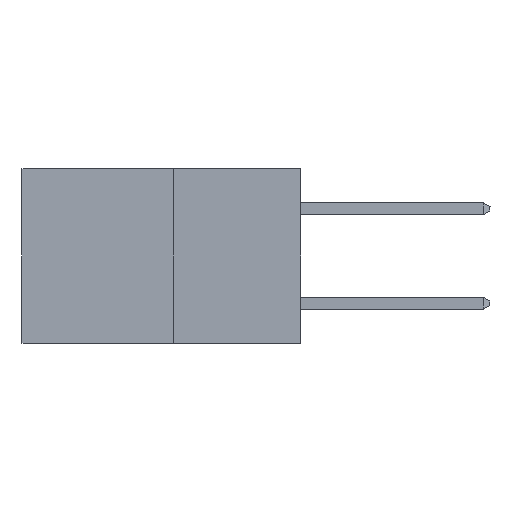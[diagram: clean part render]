
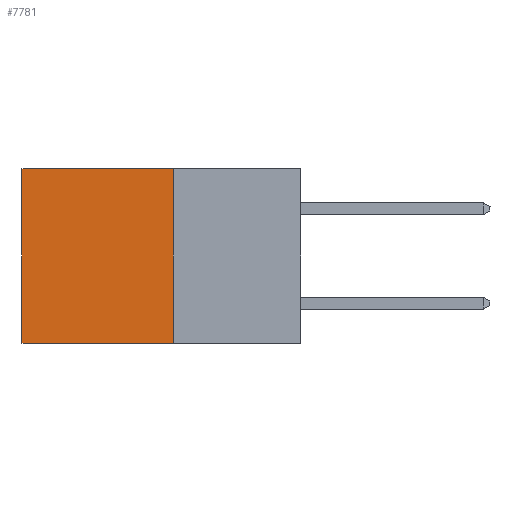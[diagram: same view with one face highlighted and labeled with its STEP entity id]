
A CAD part, left-side view. The second image highlights one B-rep face of the part: STEP entity #7781.
In plain terms, the highlighted planar face has unit normal (-1, 0, 0).
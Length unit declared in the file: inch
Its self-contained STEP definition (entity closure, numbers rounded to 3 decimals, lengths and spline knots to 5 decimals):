
#81 = EDGE_CURVE ( 'NONE', #2081, #1824, #5526, .T. ) ;
#1258 = DIRECTION ( 'NONE',  ( 0., 1., 0. ) ) ;
#1311 = LINE ( 'NONE', #8585, #3317 ) ;
#1323 = EDGE_CURVE ( 'NONE', #1824, #3009, #1311, .T. ) ;
#1560 = ORIENTED_EDGE ( 'NONE', *, *, #2377, .T. ) ;
#1824 = VERTEX_POINT ( 'NONE', #7025 ) ;
#1827 = CARTESIAN_POINT ( 'NONE',  ( 0.277, 0.59, -0.37 ) ) ;
#2081 = VERTEX_POINT ( 'NONE', #6067 ) ;
#2377 = EDGE_CURVE ( 'NONE', #9239, #3009, #8280, .T. ) ;
#2929 = CARTESIAN_POINT ( 'NONE',  ( 0.277, 0.27, 0. ) ) ;
#3009 = VERTEX_POINT ( 'NONE', #1827 ) ;
#3317 = VECTOR ( 'NONE', #9211, 39.37008 ) ;
#3790 = DIRECTION ( 'NONE',  ( 0., 0., -1. ) ) ;
#3817 = ORIENTED_EDGE ( 'NONE', *, *, #1323, .F. ) ;
#4208 = LINE ( 'NONE', #2929, #6133 ) ;
#4457 = EDGE_LOOP ( 'NONE', ( #1560, #3817, #5985, #8265 ) ) ;
#4624 = CARTESIAN_POINT ( 'NONE',  ( 0.277, 0.59, -0.37 ) ) ;
#5256 = DIRECTION ( 'NONE',  ( 0., 0., -1. ) ) ;
#5526 = LINE ( 'NONE', #5654, #9571 ) ;
#5654 = CARTESIAN_POINT ( 'NONE',  ( 0.277, 0.27, -0.37 ) ) ;
#5985 = ORIENTED_EDGE ( 'NONE', *, *, #81, .F. ) ;
#6027 = CARTESIAN_POINT ( 'NONE',  ( 0.277, 0.27, -0.37 ) ) ;
#6067 = CARTESIAN_POINT ( 'NONE',  ( 0.277, 0.27, 0. ) ) ;
#6099 = VECTOR ( 'NONE', #9314, 39.37008 ) ;
#6121 = FACE_OUTER_BOUND ( 'NONE', #4457, .T. ) ;
#6133 = VECTOR ( 'NONE', #1258, 39.37008 ) ;
#7025 = CARTESIAN_POINT ( 'NONE',  ( 0.277, 0.27, -0.37 ) ) ;
#7240 = EDGE_CURVE ( 'NONE', #2081, #9239, #4208, .T. ) ;
#7685 = PLANE ( 'NONE',  #10277 ) ;
#7781 = ADVANCED_FACE ( 'NONE', ( #6121 ), #7685, .F. ) ;
#8265 = ORIENTED_EDGE ( 'NONE', *, *, #7240, .T. ) ;
#8280 = LINE ( 'NONE', #4624, #6099 ) ;
#8585 = CARTESIAN_POINT ( 'NONE',  ( 0.277, 0.27, -0.37 ) ) ;
#9211 = DIRECTION ( 'NONE',  ( 0., 1., 0. ) ) ;
#9239 = VERTEX_POINT ( 'NONE', #9914 ) ;
#9314 = DIRECTION ( 'NONE',  ( 0., 0., -1. ) ) ;
#9571 = VECTOR ( 'NONE', #3790, 39.37008 ) ;
#9914 = CARTESIAN_POINT ( 'NONE',  ( 0.277, 0.59, 0. ) ) ;
#10056 = DIRECTION ( 'NONE',  ( 1., 0., 0. ) ) ;
#10277 = AXIS2_PLACEMENT_3D ( 'NONE', #6027, #10056, #5256 ) ;
